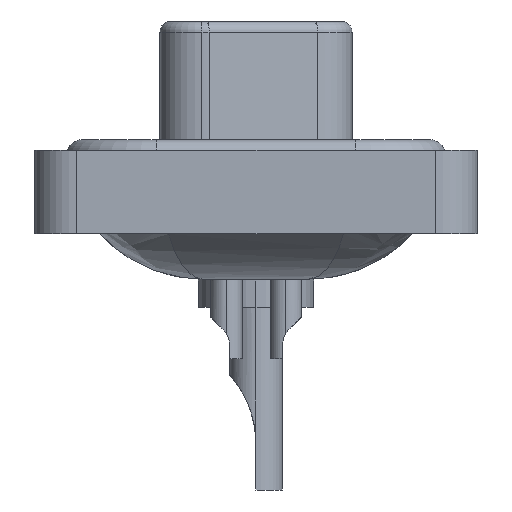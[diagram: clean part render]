
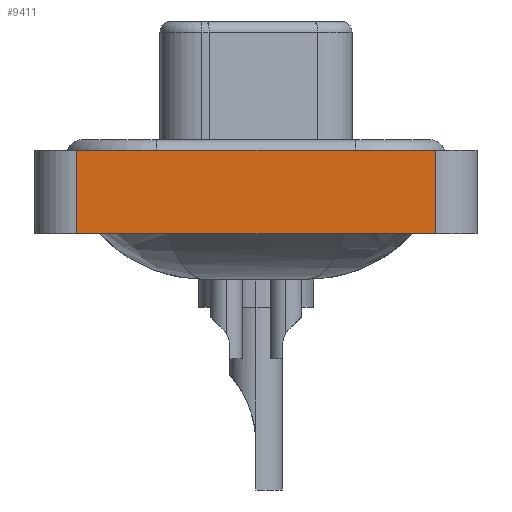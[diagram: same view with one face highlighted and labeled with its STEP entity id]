
A CAD part, left-side view. The second image highlights one B-rep face of the part: STEP entity #9411.
In plain terms, the highlighted planar face has unit normal (-1, 0, 0).
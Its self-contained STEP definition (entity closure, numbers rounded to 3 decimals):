
#587 = CARTESIAN_POINT ( 'NONE',  ( -7.35, -8.55, 0.4 ) ) ;
#1694 = DIRECTION ( 'NONE',  ( 0., -1., 0. ) ) ;
#2074 = ORIENTED_EDGE ( 'NONE', *, *, #14816, .F. ) ;
#2953 = ORIENTED_EDGE ( 'NONE', *, *, #4615, .T. ) ;
#4615 = EDGE_CURVE ( 'NONE', #21430, #10355, #9108, .T. ) ;
#4672 = AXIS2_PLACEMENT_3D ( 'NONE', #7292, #18650, #11041 ) ;
#5540 = CARTESIAN_POINT ( 'NONE',  ( -7.35, 8.55, 0.4 ) ) ;
#6714 = CARTESIAN_POINT ( 'NONE',  ( -7.35, 8.55, -3.6 ) ) ;
#6857 = DIRECTION ( 'NONE',  ( 0., 0., 1. ) ) ;
#6952 = DIRECTION ( 'NONE',  ( 0., 0., 1. ) ) ;
#7292 = CARTESIAN_POINT ( 'NONE',  ( -7.35, -8.55, -3.6 ) ) ;
#8625 = CARTESIAN_POINT ( 'NONE',  ( -7.35, -8.55, 0.4 ) ) ;
#8709 = VECTOR ( 'NONE', #6952, 1000. ) ;
#9108 = LINE ( 'NONE', #23972, #18921 ) ;
#9411 = ADVANCED_FACE ( 'NONE', ( #20520 ), #17024, .T. ) ;
#9776 = EDGE_CURVE ( 'NONE', #21318, #10355, #17745, .T. ) ;
#10355 = VERTEX_POINT ( 'NONE', #8625 ) ;
#11041 = DIRECTION ( 'NONE',  ( 0., 0., 1. ) ) ;
#12994 = EDGE_CURVE ( 'NONE', #19182, #21430, #15719, .T. ) ;
#14109 = CARTESIAN_POINT ( 'NONE',  ( -7.35, -8.55, -3.6 ) ) ;
#14816 = EDGE_CURVE ( 'NONE', #19182, #21318, #22320, .T. ) ;
#14979 = VECTOR ( 'NONE', #21880, 1000. ) ;
#15571 = CARTESIAN_POINT ( 'NONE',  ( -7.35, 8.55, -3.6 ) ) ;
#15719 = LINE ( 'NONE', #14109, #14979 ) ;
#16373 = ORIENTED_EDGE ( 'NONE', *, *, #9776, .F. ) ;
#16669 = VECTOR ( 'NONE', #1694, 1000. ) ;
#17024 = PLANE ( 'NONE',  #4672 ) ;
#17634 = CARTESIAN_POINT ( 'NONE',  ( -7.35, -8.55, -3.6 ) ) ;
#17745 = LINE ( 'NONE', #587, #16669 ) ;
#18650 = DIRECTION ( 'NONE',  ( -1., 0., 0. ) ) ;
#18921 = VECTOR ( 'NONE', #6857, 1000. ) ;
#19182 = VERTEX_POINT ( 'NONE', #15571 ) ;
#19904 = EDGE_LOOP ( 'NONE', ( #2953, #16373, #2074, #22048 ) ) ;
#20520 = FACE_OUTER_BOUND ( 'NONE', #19904, .T. ) ;
#21318 = VERTEX_POINT ( 'NONE', #5540 ) ;
#21430 = VERTEX_POINT ( 'NONE', #17634 ) ;
#21880 = DIRECTION ( 'NONE',  ( 0., -1., 0. ) ) ;
#22048 = ORIENTED_EDGE ( 'NONE', *, *, #12994, .T. ) ;
#22320 = LINE ( 'NONE', #6714, #8709 ) ;
#23972 = CARTESIAN_POINT ( 'NONE',  ( -7.35, -8.55, -3.6 ) ) ;
